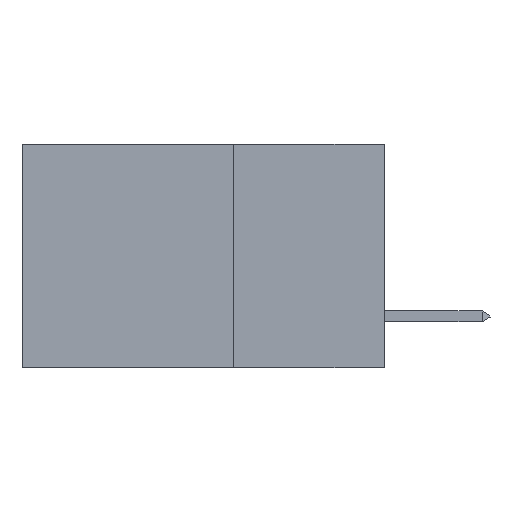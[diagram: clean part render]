
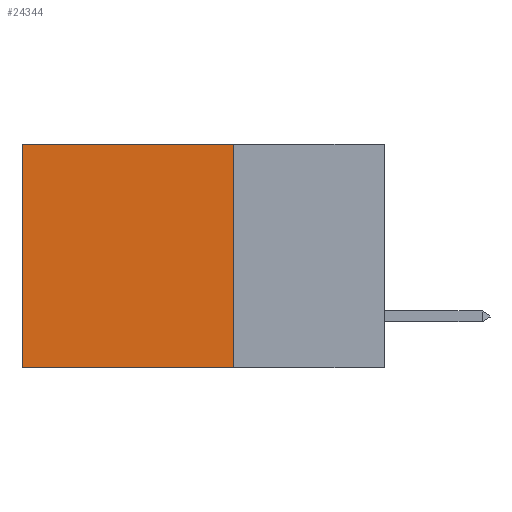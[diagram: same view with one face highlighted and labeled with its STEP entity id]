
A CAD part, left-side view. The second image highlights one B-rep face of the part: STEP entity #24344.
In plain terms, the highlighted planar face has unit normal (-1, 0, 0).
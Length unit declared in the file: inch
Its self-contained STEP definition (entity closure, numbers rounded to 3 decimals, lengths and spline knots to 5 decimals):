
#551 = CARTESIAN_POINT ( 'NONE',  ( 0.2875, 0.25, -0.37 ) ) ;
#740 = CARTESIAN_POINT ( 'NONE',  ( 0.2875, 0.25, 0. ) ) ;
#1268 = CARTESIAN_POINT ( 'NONE',  ( 0.2875, 0.6, 0. ) ) ;
#1959 = ORIENTED_EDGE ( 'NONE', *, *, #6244, .T. ) ;
#2222 = LINE ( 'NONE', #740, #33721 ) ;
#2356 = LINE ( 'NONE', #1268, #3581 ) ;
#2772 = ORIENTED_EDGE ( 'NONE', *, *, #4919, .T. ) ;
#3569 = CARTESIAN_POINT ( 'NONE',  ( 0.2875, 0.25, 0. ) ) ;
#3581 = VECTOR ( 'NONE', #22868, 39.37008 ) ;
#3915 = CARTESIAN_POINT ( 'NONE',  ( 0.2875, 0.25, -0.37 ) ) ;
#3963 = EDGE_CURVE ( 'NONE', #7156, #11979, #21270, .T. ) ;
#4166 = VERTEX_POINT ( 'NONE', #5238 ) ;
#4919 = EDGE_CURVE ( 'NONE', #4166, #9610, #2356, .T. ) ;
#5238 = CARTESIAN_POINT ( 'NONE',  ( 0.2875, 0.6, 0. ) ) ;
#5788 = DIRECTION ( 'NONE',  ( 1., 0., 0. ) ) ;
#6244 = EDGE_CURVE ( 'NONE', #7156, #4166, #2222, .T. ) ;
#6623 = ORIENTED_EDGE ( 'NONE', *, *, #8656, .F. ) ;
#7156 = VERTEX_POINT ( 'NONE', #3569 ) ;
#7540 = CARTESIAN_POINT ( 'NONE',  ( 0.2875, 0.6, -0.37 ) ) ;
#8511 = DIRECTION ( 'NONE',  ( 0., 0., -1. ) ) ;
#8656 = EDGE_CURVE ( 'NONE', #11979, #9610, #16857, .T. ) ;
#9610 = VERTEX_POINT ( 'NONE', #7540 ) ;
#11590 = CARTESIAN_POINT ( 'NONE',  ( 0.2875, 0.25, 0. ) ) ;
#11979 = VERTEX_POINT ( 'NONE', #3915 ) ;
#16857 = LINE ( 'NONE', #551, #17326 ) ;
#17326 = VECTOR ( 'NONE', #30645, 39.37008 ) ;
#19141 = CARTESIAN_POINT ( 'NONE',  ( 0.2875, 0.25, 0. ) ) ;
#20773 = EDGE_LOOP ( 'NONE', ( #2772, #6623, #33120, #1959 ) ) ;
#20858 = VECTOR ( 'NONE', #33331, 39.37008 ) ;
#21270 = LINE ( 'NONE', #11590, #20858 ) ;
#22332 = PLANE ( 'NONE',  #30538 ) ;
#22868 = DIRECTION ( 'NONE',  ( 0., 0., -1. ) ) ;
#24271 = FACE_OUTER_BOUND ( 'NONE', #20773, .T. ) ;
#24344 = ADVANCED_FACE ( 'NONE', ( #24271 ), #22332, .F. ) ;
#30308 = DIRECTION ( 'NONE',  ( 0., 1., 0. ) ) ;
#30538 = AXIS2_PLACEMENT_3D ( 'NONE', #19141, #5788, #8511 ) ;
#30645 = DIRECTION ( 'NONE',  ( 0., 1., 0. ) ) ;
#33120 = ORIENTED_EDGE ( 'NONE', *, *, #3963, .F. ) ;
#33331 = DIRECTION ( 'NONE',  ( 0., 0., -1. ) ) ;
#33721 = VECTOR ( 'NONE', #30308, 39.37008 ) ;
